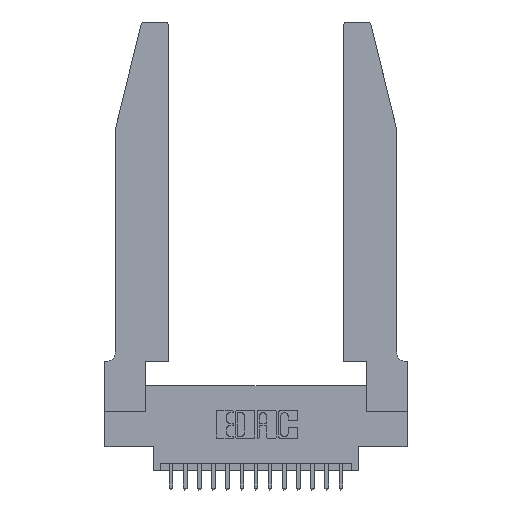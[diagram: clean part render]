
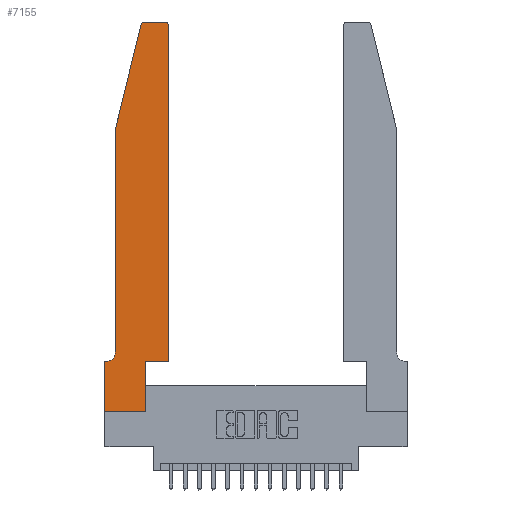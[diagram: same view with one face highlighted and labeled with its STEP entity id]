
A CAD part, top view. The second image highlights one B-rep face of the part: STEP entity #7155.
In plain terms, the highlighted planar face has unit normal (0, 0, 1).
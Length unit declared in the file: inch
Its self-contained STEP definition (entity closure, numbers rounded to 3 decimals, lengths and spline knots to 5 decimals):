
#65 = DIRECTION ( 'NONE',  ( 0., 1., 0. ) ) ;
#173 = CARTESIAN_POINT ( 'NONE',  ( 0.0755, 2., 0.37 ) ) ;
#395 = CARTESIAN_POINT ( 'NONE',  ( 0.2865, 0.35, 0.37 ) ) ;
#578 = DIRECTION ( 'NONE',  ( 0., -1., 0. ) ) ;
#728 = VECTOR ( 'NONE', #1799, 39.37008 ) ;
#1216 = CARTESIAN_POINT ( 'NONE',  ( 0.25487, 2.72718, 0.37 ) ) ;
#1227 = CARTESIAN_POINT ( 'NONE',  ( 0., 0.35, 0.37 ) ) ;
#1587 = EDGE_CURVE ( 'NONE', #17810, #10474, #9120, .T. ) ;
#1640 = CARTESIAN_POINT ( 'NONE',  ( 0.4505, 2.72, 0.37 ) ) ;
#1727 = CARTESIAN_POINT ( 'NONE',  ( 0.2865, 0., 0.37 ) ) ;
#1799 = DIRECTION ( 'NONE',  ( 1., 0., 0. ) ) ;
#2781 = DIRECTION ( 'NONE',  ( 0., 0., 1. ) ) ;
#3129 = VECTOR ( 'NONE', #16930, 39.37008 ) ;
#3138 = CARTESIAN_POINT ( 'NONE',  ( 0.4505, 0.35, 0.37 ) ) ;
#3298 = CIRCLE ( 'NONE', #9879, 0.03 ) ;
#3488 = VERTEX_POINT ( 'NONE', #14405 ) ;
#3991 = VECTOR ( 'NONE', #13182, 39.37008 ) ;
#4112 = EDGE_CURVE ( 'NONE', #14277, #18736, #4606, .T. ) ;
#4207 = EDGE_CURVE ( 'NONE', #5951, #16994, #15424, .T. ) ;
#4606 = LINE ( 'NONE', #16102, #8582 ) ;
#4683 = CIRCLE ( 'NONE', #7950, 0.03 ) ;
#4684 = LINE ( 'NONE', #14988, #728 ) ;
#4694 = DIRECTION ( 'NONE',  ( -0.239, -0.971, 0. ) ) ;
#4878 = ORIENTED_EDGE ( 'NONE', *, *, #4207, .T. ) ;
#4960 = DIRECTION ( 'NONE',  ( -1., 0., 0. ) ) ;
#5196 = VECTOR ( 'NONE', #578, 39.37008 ) ;
#5314 = VERTEX_POINT ( 'NONE', #18675 ) ;
#5451 = DIRECTION ( 'NONE',  ( 0., 0., -1. ) ) ;
#5628 = ORIENTED_EDGE ( 'NONE', *, *, #14250, .T. ) ;
#5866 = DIRECTION ( 'NONE',  ( -1., 0., 0. ) ) ;
#5928 = DIRECTION ( 'NONE',  ( 0., 0., 1. ) ) ;
#5951 = VERTEX_POINT ( 'NONE', #3138 ) ;
#6345 = EDGE_CURVE ( 'NONE', #18736, #10202, #4683, .T. ) ;
#6480 = ORIENTED_EDGE ( 'NONE', *, *, #6345, .T. ) ;
#6822 = ORIENTED_EDGE ( 'NONE', *, *, #10062, .T. ) ;
#6997 = LINE ( 'NONE', #173, #14309 ) ;
#7017 = FACE_OUTER_BOUND ( 'NONE', #9049, .T. ) ;
#7155 = ADVANCED_FACE ( 'NONE', ( #7017 ), #8721, .T. ) ;
#7295 = CARTESIAN_POINT ( 'NONE',  ( 0.0755, 2., 0.37 ) ) ;
#7553 = CARTESIAN_POINT ( 'NONE',  ( 0.4505, 0.35, 0.37 ) ) ;
#7673 = ORIENTED_EDGE ( 'NONE', *, *, #18201, .T. ) ;
#7869 = CARTESIAN_POINT ( 'NONE',  ( 0.0755, 2., 0.37 ) ) ;
#7933 = CARTESIAN_POINT ( 'NONE',  ( 0.0755, 0.42, 0.37 ) ) ;
#7950 = AXIS2_PLACEMENT_3D ( 'NONE', #8479, #18627, #9956 ) ;
#7980 = LINE ( 'NONE', #11706, #3991 ) ;
#8479 = CARTESIAN_POINT ( 'NONE',  ( 0.284, 2.72, 0.37 ) ) ;
#8582 = VECTOR ( 'NONE', #5866, 39.37008 ) ;
#8721 = PLANE ( 'NONE',  #18872 ) ;
#9049 = EDGE_LOOP ( 'NONE', ( #16900, #6480, #10456, #18283, #7673, #10731, #5628, #6822, #9914, #14882, #4878, #10295 ) ) ;
#9120 = LINE ( 'NONE', #7869, #5196 ) ;
#9250 = VERTEX_POINT ( 'NONE', #395 ) ;
#9572 = CARTESIAN_POINT ( 'NONE',  ( 0.284, 2.75, 0.37 ) ) ;
#9787 = CARTESIAN_POINT ( 'NONE',  ( 0., 0., 0.37 ) ) ;
#9879 = AXIS2_PLACEMENT_3D ( 'NONE', #14687, #5928, #16153 ) ;
#9914 = ORIENTED_EDGE ( 'NONE', *, *, #13831, .T. ) ;
#9956 = DIRECTION ( 'NONE',  ( 1., 0., 0. ) ) ;
#10062 = EDGE_CURVE ( 'NONE', #3488, #14007, #14873, .T. ) ;
#10202 = VERTEX_POINT ( 'NONE', #1216 ) ;
#10212 = VECTOR ( 'NONE', #4960, 39.37008 ) ;
#10295 = ORIENTED_EDGE ( 'NONE', *, *, #13863, .T. ) ;
#10456 = ORIENTED_EDGE ( 'NONE', *, *, #18554, .T. ) ;
#10474 = VERTEX_POINT ( 'NONE', #7933 ) ;
#10731 = ORIENTED_EDGE ( 'NONE', *, *, #15924, .T. ) ;
#11706 = CARTESIAN_POINT ( 'NONE',  ( 0.2865, 0.35, 0.37 ) ) ;
#12735 = LINE ( 'NONE', #15221, #10212 ) ;
#13123 = DIRECTION ( 'NONE',  ( 1., 0., 0. ) ) ;
#13182 = DIRECTION ( 'NONE',  ( 0., 1., 0. ) ) ;
#13680 = VECTOR ( 'NONE', #15592, 39.37008 ) ;
#13831 = EDGE_CURVE ( 'NONE', #14007, #9250, #7980, .T. ) ;
#13863 = EDGE_CURVE ( 'NONE', #16994, #14277, #3298, .T. ) ;
#14007 = VERTEX_POINT ( 'NONE', #1727 ) ;
#14044 = EDGE_CURVE ( 'NONE', #9250, #5951, #4684, .T. ) ;
#14242 = CARTESIAN_POINT ( 'NONE',  ( 0.0055, 0.42, 0.37 ) ) ;
#14250 = EDGE_CURVE ( 'NONE', #5314, #3488, #17083, .T. ) ;
#14277 = VERTEX_POINT ( 'NONE', #17099 ) ;
#14309 = VECTOR ( 'NONE', #4694, 39.37008 ) ;
#14405 = CARTESIAN_POINT ( 'NONE',  ( 0., 0., 0.37 ) ) ;
#14687 = CARTESIAN_POINT ( 'NONE',  ( 0.4205, 2.72, 0.37 ) ) ;
#14873 = LINE ( 'NONE', #15544, #3129 ) ;
#14882 = ORIENTED_EDGE ( 'NONE', *, *, #14044, .T. ) ;
#14988 = CARTESIAN_POINT ( 'NONE',  ( 0.4505, 0.35, 0.37 ) ) ;
#15221 = CARTESIAN_POINT ( 'NONE',  ( 0.0755, 0.35, 0.37 ) ) ;
#15424 = LINE ( 'NONE', #7553, #18337 ) ;
#15544 = CARTESIAN_POINT ( 'NONE',  ( 0., 0., 0.37 ) ) ;
#15592 = DIRECTION ( 'NONE',  ( 0., -1., 0. ) ) ;
#15716 = DIRECTION ( 'NONE',  ( -1., 0., 0. ) ) ;
#15924 = EDGE_CURVE ( 'NONE', #19005, #5314, #12735, .T. ) ;
#16102 = CARTESIAN_POINT ( 'NONE',  ( 0.2605, 2.75, 0.37 ) ) ;
#16153 = DIRECTION ( 'NONE',  ( 1., 0., 0. ) ) ;
#16356 = CIRCLE ( 'NONE', #17811, 0.07 ) ;
#16900 = ORIENTED_EDGE ( 'NONE', *, *, #4112, .T. ) ;
#16930 = DIRECTION ( 'NONE',  ( 1., 0., 0. ) ) ;
#16994 = VERTEX_POINT ( 'NONE', #1640 ) ;
#17083 = LINE ( 'NONE', #9787, #13680 ) ;
#17099 = CARTESIAN_POINT ( 'NONE',  ( 0.4205, 2.75, 0.37 ) ) ;
#17566 = CARTESIAN_POINT ( 'NONE',  ( 0.0055, 0.35, 0.37 ) ) ;
#17810 = VERTEX_POINT ( 'NONE', #7295 ) ;
#17811 = AXIS2_PLACEMENT_3D ( 'NONE', #14242, #5451, #15716 ) ;
#18201 = EDGE_CURVE ( 'NONE', #10474, #19005, #16356, .T. ) ;
#18283 = ORIENTED_EDGE ( 'NONE', *, *, #1587, .T. ) ;
#18337 = VECTOR ( 'NONE', #65, 39.37008 ) ;
#18554 = EDGE_CURVE ( 'NONE', #10202, #17810, #6997, .T. ) ;
#18627 = DIRECTION ( 'NONE',  ( 0., 0., 1. ) ) ;
#18675 = CARTESIAN_POINT ( 'NONE',  ( 0., 0.35, 0.37 ) ) ;
#18736 = VERTEX_POINT ( 'NONE', #9572 ) ;
#18872 = AXIS2_PLACEMENT_3D ( 'NONE', #1227, #2781, #13123 ) ;
#19005 = VERTEX_POINT ( 'NONE', #17566 ) ;
